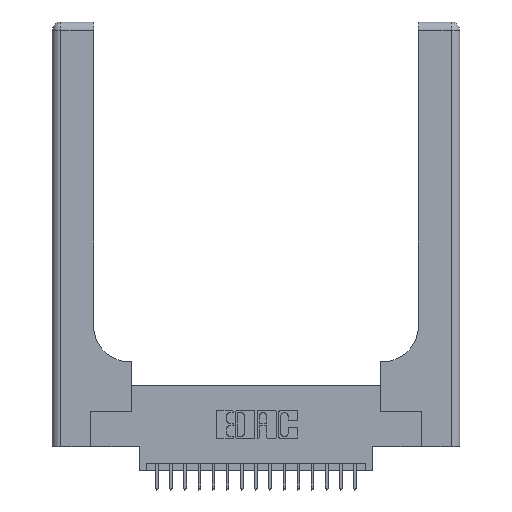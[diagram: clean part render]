
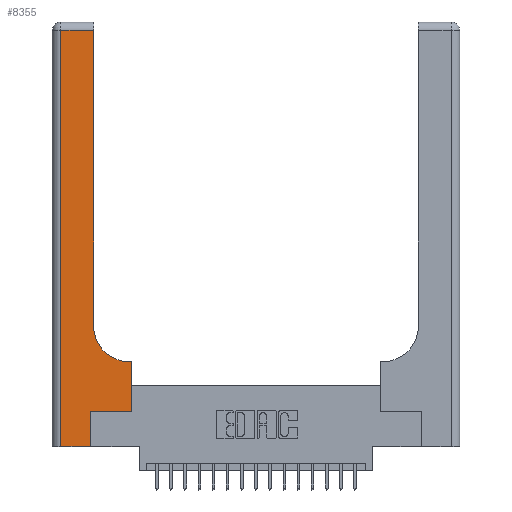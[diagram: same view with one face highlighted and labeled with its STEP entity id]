
A CAD part, top view. The second image highlights one B-rep face of the part: STEP entity #8355.
In plain terms, the highlighted planar face has unit normal (0, 0, 1).
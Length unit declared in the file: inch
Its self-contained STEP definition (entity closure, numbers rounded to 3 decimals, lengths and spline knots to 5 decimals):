
#105 = EDGE_CURVE ( 'NONE', #7808, #18630, #10727, .T. ) ;
#264 = CARTESIAN_POINT ( 'NONE',  ( 0., 2.94, 0.37 ) ) ;
#818 = DIRECTION ( 'NONE',  ( 0., 1., 0. ) ) ;
#901 = DIRECTION ( 'NONE',  ( 0., 1., 0. ) ) ;
#926 = VECTOR ( 'NONE', #17892, 39.37008 ) ;
#1734 = CARTESIAN_POINT ( 'NONE',  ( 0., 0., 0.37 ) ) ;
#1896 = VERTEX_POINT ( 'NONE', #2213 ) ;
#2213 = CARTESIAN_POINT ( 'NONE',  ( 0.06, 0., 0.37 ) ) ;
#2723 = DIRECTION ( 'NONE',  ( -1., 0., 0. ) ) ;
#2814 = CARTESIAN_POINT ( 'NONE',  ( 0.2915, 0.6, 0.37 ) ) ;
#3114 = DIRECTION ( 'NONE',  ( 0., -1., 0. ) ) ;
#3296 = VERTEX_POINT ( 'NONE', #10287 ) ;
#3640 = CARTESIAN_POINT ( 'NONE',  ( 0.2915, 2.94, 0.37 ) ) ;
#3688 = CARTESIAN_POINT ( 'NONE',  ( 0.269, 0., 0.37 ) ) ;
#4080 = LINE ( 'NONE', #13894, #15061 ) ;
#4122 = VERTEX_POINT ( 'NONE', #16822 ) ;
#6347 = EDGE_CURVE ( 'NONE', #18630, #15990, #11105, .T. ) ;
#6366 = VERTEX_POINT ( 'NONE', #3688 ) ;
#6377 = DIRECTION ( 'NONE',  ( -1., 0., 0. ) ) ;
#6380 = LINE ( 'NONE', #7818, #10508 ) ;
#6532 = CARTESIAN_POINT ( 'NONE',  ( 0.5415, 0.85, 0.37 ) ) ;
#6585 = CARTESIAN_POINT ( 'NONE',  ( 0., 3., 0.37 ) ) ;
#7406 = CARTESIAN_POINT ( 'NONE',  ( 0.269, 0., 0.37 ) ) ;
#7808 = VERTEX_POINT ( 'NONE', #15986 ) ;
#7818 = CARTESIAN_POINT ( 'NONE',  ( 0.269, 0.25, 0.37 ) ) ;
#8162 = AXIS2_PLACEMENT_3D ( 'NONE', #6585, #19089, #14438 ) ;
#8335 = EDGE_CURVE ( 'NONE', #4122, #17254, #6380, .T. ) ;
#8355 = ADVANCED_FACE ( 'NONE', ( #17722 ), #15827, .F. ) ;
#8667 = CARTESIAN_POINT ( 'NONE',  ( 0.5415, 0.6, 0.37 ) ) ;
#8819 = CARTESIAN_POINT ( 'NONE',  ( 0.5585, 0.25, 0.37 ) ) ;
#8850 = ORIENTED_EDGE ( 'NONE', *, *, #15763, .T. ) ;
#9152 = ORIENTED_EDGE ( 'NONE', *, *, #11032, .T. ) ;
#9256 = CARTESIAN_POINT ( 'NONE',  ( 0.2915, 0.85, 0.37 ) ) ;
#9728 = ORIENTED_EDGE ( 'NONE', *, *, #6347, .T. ) ;
#9796 = AXIS2_PLACEMENT_3D ( 'NONE', #6532, #12877, #17767 ) ;
#10277 = LINE ( 'NONE', #16510, #19021 ) ;
#10287 = CARTESIAN_POINT ( 'NONE',  ( 0.06, 2.94, 0.37 ) ) ;
#10508 = VECTOR ( 'NONE', #16040, 39.37008 ) ;
#10613 = VECTOR ( 'NONE', #3114, 39.37008 ) ;
#10702 = EDGE_LOOP ( 'NONE', ( #10743, #13906, #11077, #11549, #8850, #12241, #9152, #20116, #9728 ) ) ;
#10727 = LINE ( 'NONE', #2814, #16909 ) ;
#10743 = ORIENTED_EDGE ( 'NONE', *, *, #15467, .T. ) ;
#11032 = EDGE_CURVE ( 'NONE', #17254, #7808, #10277, .T. ) ;
#11077 = ORIENTED_EDGE ( 'NONE', *, *, #11754, .T. ) ;
#11105 = CIRCLE ( 'NONE', #9796, 0.25 ) ;
#11549 = ORIENTED_EDGE ( 'NONE', *, *, #11844, .T. ) ;
#11754 = EDGE_CURVE ( 'NONE', #3296, #1896, #19064, .T. ) ;
#11844 = EDGE_CURVE ( 'NONE', #1896, #6366, #16114, .T. ) ;
#11960 = VECTOR ( 'NONE', #6377, 39.37008 ) ;
#12241 = ORIENTED_EDGE ( 'NONE', *, *, #8335, .T. ) ;
#12482 = EDGE_CURVE ( 'NONE', #17424, #3296, #18798, .T. ) ;
#12877 = DIRECTION ( 'NONE',  ( 0., 0., -1. ) ) ;
#13770 = LINE ( 'NONE', #7406, #18411 ) ;
#13894 = CARTESIAN_POINT ( 'NONE',  ( 0.2915, 3., 0.37 ) ) ;
#13906 = ORIENTED_EDGE ( 'NONE', *, *, #12482, .T. ) ;
#14438 = DIRECTION ( 'NONE',  ( -1., 0., 0. ) ) ;
#15061 = VECTOR ( 'NONE', #818, 39.37008 ) ;
#15467 = EDGE_CURVE ( 'NONE', #15990, #17424, #4080, .T. ) ;
#15763 = EDGE_CURVE ( 'NONE', #6366, #4122, #13770, .T. ) ;
#15800 = CARTESIAN_POINT ( 'NONE',  ( 0.06, 3., 0.37 ) ) ;
#15827 = PLANE ( 'NONE',  #8162 ) ;
#15986 = CARTESIAN_POINT ( 'NONE',  ( 0.5585, 0.6, 0.37 ) ) ;
#15990 = VERTEX_POINT ( 'NONE', #9256 ) ;
#16040 = DIRECTION ( 'NONE',  ( 1., 0., 0. ) ) ;
#16114 = LINE ( 'NONE', #1734, #926 ) ;
#16510 = CARTESIAN_POINT ( 'NONE',  ( 0.5585, 0.25, 0.37 ) ) ;
#16822 = CARTESIAN_POINT ( 'NONE',  ( 0.269, 0.25, 0.37 ) ) ;
#16909 = VECTOR ( 'NONE', #2723, 39.37008 ) ;
#17254 = VERTEX_POINT ( 'NONE', #8819 ) ;
#17424 = VERTEX_POINT ( 'NONE', #3640 ) ;
#17722 = FACE_OUTER_BOUND ( 'NONE', #10702, .T. ) ;
#17767 = DIRECTION ( 'NONE',  ( 1., 0., 0. ) ) ;
#17892 = DIRECTION ( 'NONE',  ( 1., 0., 0. ) ) ;
#18411 = VECTOR ( 'NONE', #901, 39.37008 ) ;
#18630 = VERTEX_POINT ( 'NONE', #8667 ) ;
#18798 = LINE ( 'NONE', #264, #11960 ) ;
#19021 = VECTOR ( 'NONE', #19580, 39.37008 ) ;
#19064 = LINE ( 'NONE', #15800, #10613 ) ;
#19089 = DIRECTION ( 'NONE',  ( 0., 0., -1. ) ) ;
#19580 = DIRECTION ( 'NONE',  ( 0., 1., 0. ) ) ;
#20116 = ORIENTED_EDGE ( 'NONE', *, *, #105, .T. ) ;
